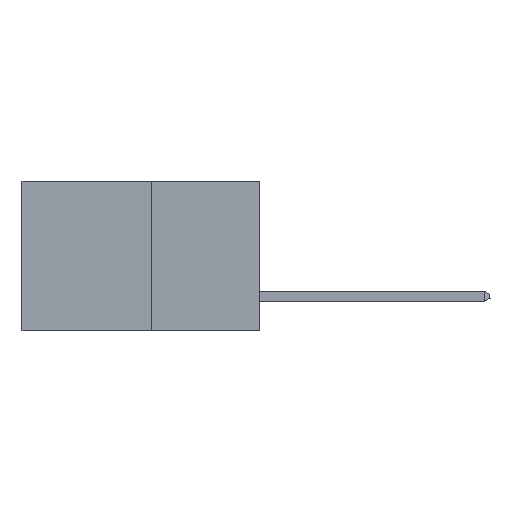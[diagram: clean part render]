
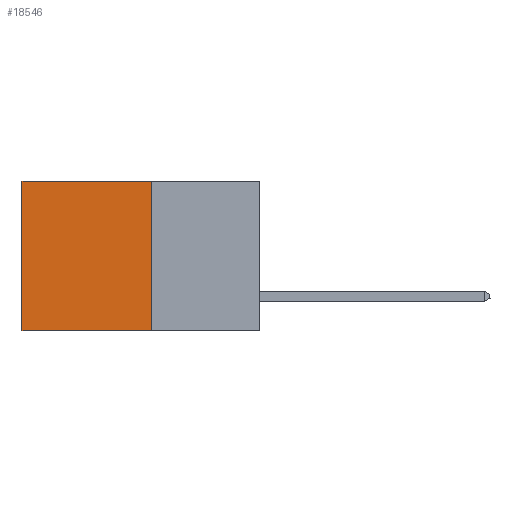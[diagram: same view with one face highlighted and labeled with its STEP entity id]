
A CAD part, left-side view. The second image highlights one B-rep face of the part: STEP entity #18546.
In plain terms, the highlighted planar face has unit normal (-1, 0, 0).
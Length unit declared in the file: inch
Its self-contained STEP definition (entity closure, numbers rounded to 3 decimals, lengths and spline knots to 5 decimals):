
#673 = DIRECTION ( 'NONE',  ( 0., 1., 0. ) ) ;
#797 = DIRECTION ( 'NONE',  ( 0., 0., -1. ) ) ;
#884 = CARTESIAN_POINT ( 'NONE',  ( 0.277, 0.27, 0. ) ) ;
#1496 = CARTESIAN_POINT ( 'NONE',  ( 0.277, 0.27, -0.37 ) ) ;
#2216 = AXIS2_PLACEMENT_3D ( 'NONE', #19537, #9605, #21214 ) ;
#2291 = EDGE_CURVE ( 'NONE', #8529, #6040, #13386, .T. ) ;
#2925 = EDGE_LOOP ( 'NONE', ( #13510, #21264, #20646, #4022 ) ) ;
#4022 = ORIENTED_EDGE ( 'NONE', *, *, #11231, .T. ) ;
#4452 = CARTESIAN_POINT ( 'NONE',  ( 0.277, 0.27, -0.37 ) ) ;
#4757 = VECTOR ( 'NONE', #13050, 39.37008 ) ;
#5712 = CARTESIAN_POINT ( 'NONE',  ( 0.277, 0.59, -0.37 ) ) ;
#6040 = VERTEX_POINT ( 'NONE', #6301 ) ;
#6301 = CARTESIAN_POINT ( 'NONE',  ( 0.277, 0.59, -0.37 ) ) ;
#8529 = VERTEX_POINT ( 'NONE', #20315 ) ;
#8649 = LINE ( 'NONE', #1496, #4757 ) ;
#8730 = CARTESIAN_POINT ( 'NONE',  ( 0.277, 0.59, 0. ) ) ;
#8979 = VECTOR ( 'NONE', #20961, 39.37008 ) ;
#9311 = VERTEX_POINT ( 'NONE', #884 ) ;
#9605 = DIRECTION ( 'NONE',  ( 1., 0., 0. ) ) ;
#10471 = VECTOR ( 'NONE', #673, 39.37008 ) ;
#10622 = VERTEX_POINT ( 'NONE', #8730 ) ;
#10882 = EDGE_CURVE ( 'NONE', #9311, #8529, #8649, .T. ) ;
#11231 = EDGE_CURVE ( 'NONE', #9311, #10622, #19796, .T. ) ;
#12884 = FACE_OUTER_BOUND ( 'NONE', #2925, .T. ) ;
#13050 = DIRECTION ( 'NONE',  ( 0., 0., -1. ) ) ;
#13386 = LINE ( 'NONE', #4452, #8979 ) ;
#13510 = ORIENTED_EDGE ( 'NONE', *, *, #14540, .T. ) ;
#13923 = CARTESIAN_POINT ( 'NONE',  ( 0.277, 0.27, 0. ) ) ;
#14540 = EDGE_CURVE ( 'NONE', #10622, #6040, #21198, .T. ) ;
#16830 = VECTOR ( 'NONE', #797, 39.37008 ) ;
#18546 = ADVANCED_FACE ( 'NONE', ( #12884 ), #21140, .F. ) ;
#19537 = CARTESIAN_POINT ( 'NONE',  ( 0.277, 0.27, -0.37 ) ) ;
#19796 = LINE ( 'NONE', #13923, #10471 ) ;
#20315 = CARTESIAN_POINT ( 'NONE',  ( 0.277, 0.27, -0.37 ) ) ;
#20646 = ORIENTED_EDGE ( 'NONE', *, *, #10882, .F. ) ;
#20961 = DIRECTION ( 'NONE',  ( 0., 1., 0. ) ) ;
#21140 = PLANE ( 'NONE',  #2216 ) ;
#21198 = LINE ( 'NONE', #5712, #16830 ) ;
#21214 = DIRECTION ( 'NONE',  ( 0., 0., -1. ) ) ;
#21264 = ORIENTED_EDGE ( 'NONE', *, *, #2291, .F. ) ;
